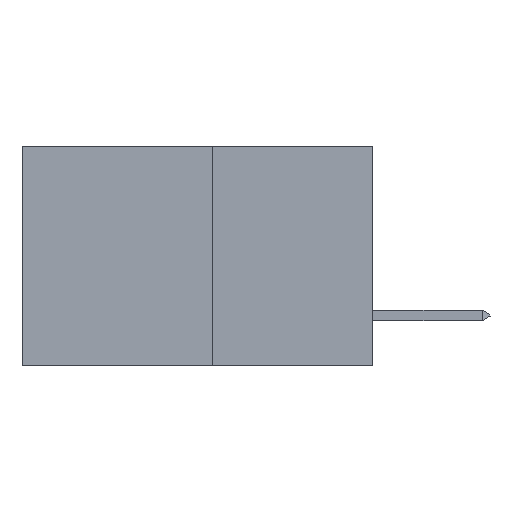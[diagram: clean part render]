
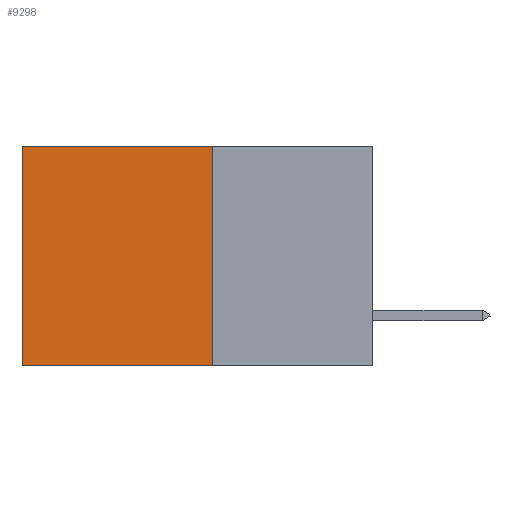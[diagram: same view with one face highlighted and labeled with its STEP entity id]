
A CAD part, left-side view. The second image highlights one B-rep face of the part: STEP entity #9298.
In plain terms, the highlighted planar face has unit normal (-1, 0, 0).
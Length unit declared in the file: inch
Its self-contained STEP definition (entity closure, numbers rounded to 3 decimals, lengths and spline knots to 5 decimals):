
#324 = CARTESIAN_POINT ( 'NONE',  ( 0.277, 0.27, -0.37 ) ) ;
#1112 = LINE ( 'NONE', #9924, #13156 ) ;
#1113 = DIRECTION ( 'NONE',  ( 0., 0., -1. ) ) ;
#2899 = CARTESIAN_POINT ( 'NONE',  ( 0.277, 0.27, -0.37 ) ) ;
#3471 = PLANE ( 'NONE',  #13105 ) ;
#3478 = VECTOR ( 'NONE', #1113, 39.37008 ) ;
#4050 = EDGE_CURVE ( 'NONE', #6308, #12386, #1112, .T. ) ;
#4154 = ORIENTED_EDGE ( 'NONE', *, *, #4050, .F. ) ;
#6308 = VERTEX_POINT ( 'NONE', #2899 ) ;
#6643 = EDGE_CURVE ( 'NONE', #8810, #12386, #17188, .T. ) ;
#6648 = DIRECTION ( 'NONE',  ( 0., 0., -1. ) ) ;
#6725 = CARTESIAN_POINT ( 'NONE',  ( 0.277, 0.59, 0. ) ) ;
#8006 = CARTESIAN_POINT ( 'NONE',  ( 0.277, 0.27, 0. ) ) ;
#8113 = VERTEX_POINT ( 'NONE', #15667 ) ;
#8616 = VECTOR ( 'NONE', #11638, 39.37008 ) ;
#8810 = VERTEX_POINT ( 'NONE', #6725 ) ;
#9298 = ADVANCED_FACE ( 'NONE', ( #17058 ), #3471, .F. ) ;
#9643 = DIRECTION ( 'NONE',  ( 0., 1., 0. ) ) ;
#9721 = LINE ( 'NONE', #8006, #17743 ) ;
#9924 = CARTESIAN_POINT ( 'NONE',  ( 0.277, 0.27, -0.37 ) ) ;
#9983 = DIRECTION ( 'NONE',  ( 0., 1., 0. ) ) ;
#10062 = CARTESIAN_POINT ( 'NONE',  ( 0.277, 0.59, -0.37 ) ) ;
#11566 = ORIENTED_EDGE ( 'NONE', *, *, #6643, .T. ) ;
#11638 = DIRECTION ( 'NONE',  ( 0., 0., -1. ) ) ;
#12150 = CARTESIAN_POINT ( 'NONE',  ( 0.277, 0.59, -0.37 ) ) ;
#12386 = VERTEX_POINT ( 'NONE', #12150 ) ;
#12543 = ORIENTED_EDGE ( 'NONE', *, *, #17557, .F. ) ;
#13105 = AXIS2_PLACEMENT_3D ( 'NONE', #324, #15872, #6648 ) ;
#13156 = VECTOR ( 'NONE', #9983, 39.37008 ) ;
#15667 = CARTESIAN_POINT ( 'NONE',  ( 0.277, 0.27, 0. ) ) ;
#15848 = LINE ( 'NONE', #19523, #3478 ) ;
#15872 = DIRECTION ( 'NONE',  ( 1., 0., 0. ) ) ;
#16562 = EDGE_CURVE ( 'NONE', #8113, #8810, #9721, .T. ) ;
#17058 = FACE_OUTER_BOUND ( 'NONE', #17962, .T. ) ;
#17188 = LINE ( 'NONE', #10062, #8616 ) ;
#17557 = EDGE_CURVE ( 'NONE', #8113, #6308, #15848, .T. ) ;
#17743 = VECTOR ( 'NONE', #9643, 39.37008 ) ;
#17858 = ORIENTED_EDGE ( 'NONE', *, *, #16562, .T. ) ;
#17962 = EDGE_LOOP ( 'NONE', ( #11566, #4154, #12543, #17858 ) ) ;
#19523 = CARTESIAN_POINT ( 'NONE',  ( 0.277, 0.27, -0.37 ) ) ;
